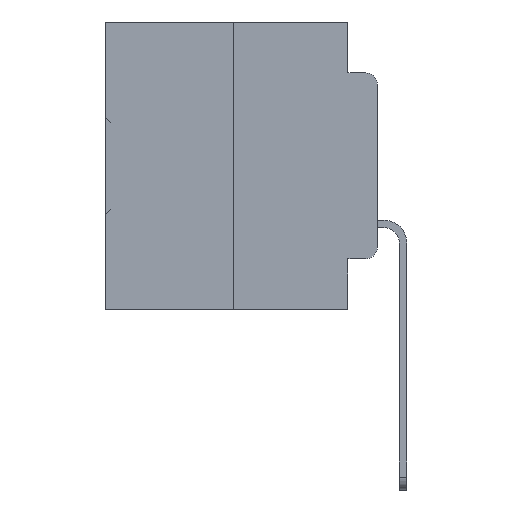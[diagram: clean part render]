
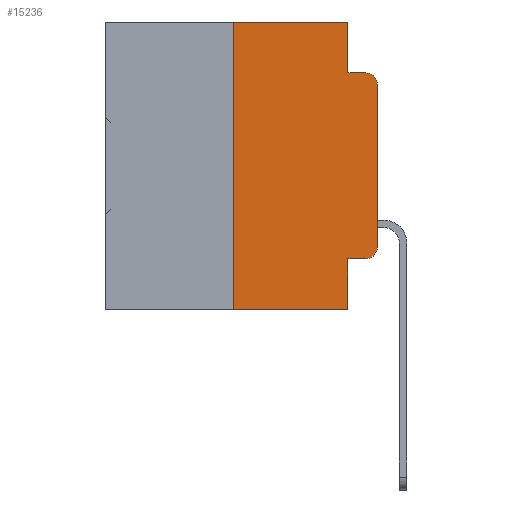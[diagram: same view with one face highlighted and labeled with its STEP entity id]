
A CAD part, left-side view. The second image highlights one B-rep face of the part: STEP entity #15236.
In plain terms, the highlighted planar face has unit normal (-1, 0, 0).
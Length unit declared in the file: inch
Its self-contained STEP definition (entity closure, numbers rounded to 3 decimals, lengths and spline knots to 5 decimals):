
#352 = DIRECTION ( 'NONE',  ( 0., 0., -1. ) ) ;
#530 = VECTOR ( 'NONE', #35896, 39.37008 ) ;
#1369 = ORIENTED_EDGE ( 'NONE', *, *, #30189, .T. ) ;
#1406 = CARTESIAN_POINT ( 'NONE',  ( 0., 0.051, -0.0885 ) ) ;
#1518 = EDGE_CURVE ( 'NONE', #20894, #33866, #12101, .T. ) ;
#1863 = ORIENTED_EDGE ( 'NONE', *, *, #23618, .T. ) ;
#1960 = CARTESIAN_POINT ( 'NONE',  ( 0., 0.051, 0. ) ) ;
#2960 = ORIENTED_EDGE ( 'NONE', *, *, #14044, .F. ) ;
#4223 = DIRECTION ( 'NONE',  ( 1., 0., 0. ) ) ;
#4535 = VECTOR ( 'NONE', #23710, 39.37008 ) ;
#5004 = VECTOR ( 'NONE', #26048, 39.37008 ) ;
#5196 = AXIS2_PLACEMENT_3D ( 'NONE', #11536, #25594, #8574 ) ;
#5850 = AXIS2_PLACEMENT_3D ( 'NONE', #23874, #4223, #7097 ) ;
#6535 = EDGE_CURVE ( 'NONE', #27352, #28833, #32632, .T. ) ;
#6675 = CARTESIAN_POINT ( 'NONE',  ( 0., 0., -0.3915 ) ) ;
#6879 = LINE ( 'NONE', #30247, #36220 ) ;
#7094 = VERTEX_POINT ( 'NONE', #31966 ) ;
#7097 = DIRECTION ( 'NONE',  ( 0., 0., -1. ) ) ;
#7102 = CIRCLE ( 'NONE', #29602, 0.02 ) ;
#7226 = CARTESIAN_POINT ( 'NONE',  ( 0., 0.051, -0.4115 ) ) ;
#8136 = VERTEX_POINT ( 'NONE', #15004 ) ;
#8200 = DIRECTION ( 'NONE',  ( -1., 0., 0. ) ) ;
#8279 = ORIENTED_EDGE ( 'NONE', *, *, #1518, .T. ) ;
#8574 = DIRECTION ( 'NONE',  ( 0., 0., -1. ) ) ;
#9673 = EDGE_CURVE ( 'NONE', #22144, #7094, #27448, .T. ) ;
#9956 = VECTOR ( 'NONE', #25916, 39.37008 ) ;
#10179 = CARTESIAN_POINT ( 'NONE',  ( 0., 0.25, 0. ) ) ;
#10724 = VERTEX_POINT ( 'NONE', #6675 ) ;
#11536 = CARTESIAN_POINT ( 'NONE',  ( 0., 0.02, -0.1085 ) ) ;
#12101 = LINE ( 'NONE', #34259, #5004 ) ;
#13760 = ORIENTED_EDGE ( 'NONE', *, *, #17793, .T. ) ;
#14044 = EDGE_CURVE ( 'NONE', #20894, #22670, #24575, .T. ) ;
#14164 = CARTESIAN_POINT ( 'NONE',  ( 0., 0.473, -0.5 ) ) ;
#14425 = VERTEX_POINT ( 'NONE', #16493 ) ;
#14748 = CARTESIAN_POINT ( 'NONE',  ( 0., 0.473, 0. ) ) ;
#15004 = CARTESIAN_POINT ( 'NONE',  ( 0., 0.25, -0.5 ) ) ;
#15083 = EDGE_CURVE ( 'NONE', #28833, #22144, #19665, .T. ) ;
#15236 = ADVANCED_FACE ( 'NONE', ( #32948 ), #26586, .F. ) ;
#15666 = LINE ( 'NONE', #10179, #530 ) ;
#15979 = CARTESIAN_POINT ( 'NONE',  ( 0., 0.051, -0.5 ) ) ;
#16493 = CARTESIAN_POINT ( 'NONE',  ( 0., 0., -0.1085 ) ) ;
#17209 = VECTOR ( 'NONE', #30526, 39.37008 ) ;
#17403 = CARTESIAN_POINT ( 'NONE',  ( 0., 0.25, 0. ) ) ;
#17793 = EDGE_CURVE ( 'NONE', #14425, #7094, #28744, .T. ) ;
#17878 = CARTESIAN_POINT ( 'NONE',  ( 0., 0.051, 0. ) ) ;
#18236 = VECTOR ( 'NONE', #22595, 39.37008 ) ;
#19665 = LINE ( 'NONE', #22632, #33873 ) ;
#20353 = EDGE_CURVE ( 'NONE', #10724, #14425, #6879, .T. ) ;
#20879 = ORIENTED_EDGE ( 'NONE', *, *, #15083, .F. ) ;
#20894 = VERTEX_POINT ( 'NONE', #7226 ) ;
#21233 = EDGE_LOOP ( 'NONE', ( #30020, #13760, #26381, #20879, #29396, #27740, #1863, #2960, #8279, #1369 ) ) ;
#21563 = DIRECTION ( 'NONE',  ( 0., 0., 1. ) ) ;
#22144 = VERTEX_POINT ( 'NONE', #1406 ) ;
#22595 = DIRECTION ( 'NONE',  ( 0., -1., 0. ) ) ;
#22632 = CARTESIAN_POINT ( 'NONE',  ( 0., 0.051, 0. ) ) ;
#22670 = VERTEX_POINT ( 'NONE', #15979 ) ;
#23618 = EDGE_CURVE ( 'NONE', #8136, #22670, #33781, .T. ) ;
#23710 = DIRECTION ( 'NONE',  ( 0., 0., -1. ) ) ;
#23874 = CARTESIAN_POINT ( 'NONE',  ( 0., 0.473, 0. ) ) ;
#24575 = LINE ( 'NONE', #17878, #4535 ) ;
#25343 = DIRECTION ( 'NONE',  ( 0., 0., -1. ) ) ;
#25594 = DIRECTION ( 'NONE',  ( -1., 0., 0. ) ) ;
#25916 = DIRECTION ( 'NONE',  ( 0., -1., 0. ) ) ;
#26048 = DIRECTION ( 'NONE',  ( 0., -1., 0. ) ) ;
#26381 = ORIENTED_EDGE ( 'NONE', *, *, #9673, .F. ) ;
#26586 = PLANE ( 'NONE',  #5850 ) ;
#27352 = VERTEX_POINT ( 'NONE', #17403 ) ;
#27448 = LINE ( 'NONE', #27793, #17209 ) ;
#27740 = ORIENTED_EDGE ( 'NONE', *, *, #28839, .F. ) ;
#27793 = CARTESIAN_POINT ( 'NONE',  ( 0., 0.051, -0.0885 ) ) ;
#28318 = CARTESIAN_POINT ( 'NONE',  ( 0., 0.02, -0.3915 ) ) ;
#28744 = CIRCLE ( 'NONE', #5196, 0.02 ) ;
#28833 = VERTEX_POINT ( 'NONE', #1960 ) ;
#28839 = EDGE_CURVE ( 'NONE', #8136, #27352, #15666, .T. ) ;
#29337 = CARTESIAN_POINT ( 'NONE',  ( 0., 0.02, -0.4115 ) ) ;
#29396 = ORIENTED_EDGE ( 'NONE', *, *, #6535, .F. ) ;
#29602 = AXIS2_PLACEMENT_3D ( 'NONE', #28318, #8200, #25343 ) ;
#30020 = ORIENTED_EDGE ( 'NONE', *, *, #20353, .T. ) ;
#30189 = EDGE_CURVE ( 'NONE', #33866, #10724, #7102, .T. ) ;
#30247 = CARTESIAN_POINT ( 'NONE',  ( 0., 0., 0. ) ) ;
#30526 = DIRECTION ( 'NONE',  ( 0., -1., 0. ) ) ;
#31966 = CARTESIAN_POINT ( 'NONE',  ( 0., 0.02, -0.0885 ) ) ;
#32632 = LINE ( 'NONE', #14748, #9956 ) ;
#32948 = FACE_OUTER_BOUND ( 'NONE', #21233, .T. ) ;
#33781 = LINE ( 'NONE', #14164, #18236 ) ;
#33866 = VERTEX_POINT ( 'NONE', #29337 ) ;
#33873 = VECTOR ( 'NONE', #352, 39.37008 ) ;
#34259 = CARTESIAN_POINT ( 'NONE',  ( 0., 0.051, -0.4115 ) ) ;
#35896 = DIRECTION ( 'NONE',  ( 0., 0., 1. ) ) ;
#36220 = VECTOR ( 'NONE', #21563, 39.37008 ) ;
